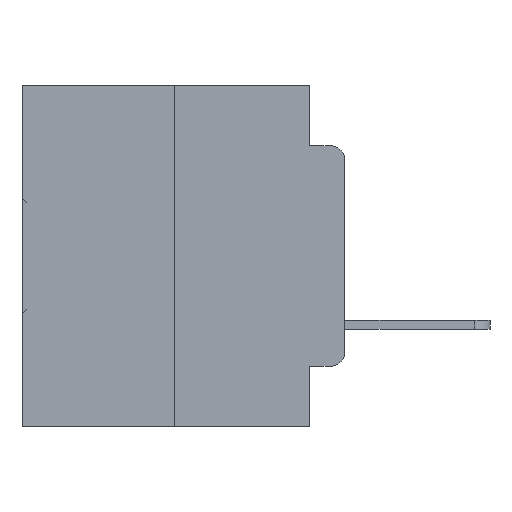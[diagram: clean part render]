
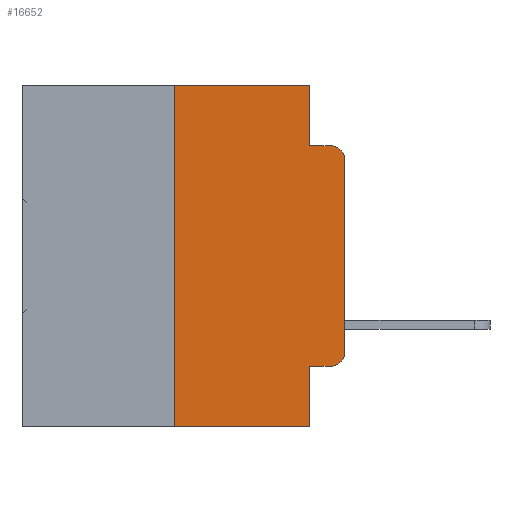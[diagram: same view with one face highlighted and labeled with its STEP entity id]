
A CAD part, left-side view. The second image highlights one B-rep face of the part: STEP entity #16652.
In plain terms, the highlighted planar face has unit normal (-1, 0, 0).
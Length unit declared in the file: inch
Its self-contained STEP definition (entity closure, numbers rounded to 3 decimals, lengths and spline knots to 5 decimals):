
#657 = AXIS2_PLACEMENT_3D ( 'NONE', #22815, #7320, #25339 ) ;
#682 = CARTESIAN_POINT ( 'NONE',  ( 0., 0., -0.1085 ) ) ;
#2944 = DIRECTION ( 'NONE',  ( 0., 0., -1. ) ) ;
#2986 = CARTESIAN_POINT ( 'NONE',  ( 0., 0.473, -0.5 ) ) ;
#3267 = VERTEX_POINT ( 'NONE', #15099 ) ;
#3400 = CARTESIAN_POINT ( 'NONE',  ( 0., 0.25, 0. ) ) ;
#3651 = ORIENTED_EDGE ( 'NONE', *, *, #21678, .F. ) ;
#3696 = PLANE ( 'NONE',  #26915 ) ;
#4369 = VERTEX_POINT ( 'NONE', #7891 ) ;
#4534 = LINE ( 'NONE', #17505, #10753 ) ;
#5088 = CARTESIAN_POINT ( 'NONE',  ( 0., 0.02, -0.4115 ) ) ;
#5525 = LINE ( 'NONE', #22235, #31099 ) ;
#5528 = DIRECTION ( 'NONE',  ( -1., 0., 0. ) ) ;
#5953 = AXIS2_PLACEMENT_3D ( 'NONE', #21174, #5528, #23659 ) ;
#5963 = EDGE_CURVE ( 'NONE', #14228, #21181, #8022, .T. ) ;
#6671 = DIRECTION ( 'NONE',  ( 0., -1., 0. ) ) ;
#7320 = DIRECTION ( 'NONE',  ( -1., 0., 0. ) ) ;
#7891 = CARTESIAN_POINT ( 'NONE',  ( 0., 0.051, -0.0885 ) ) ;
#7897 = DIRECTION ( 'NONE',  ( 0., -1., 0. ) ) ;
#8022 = LINE ( 'NONE', #25856, #21050 ) ;
#8252 = ORIENTED_EDGE ( 'NONE', *, *, #31613, .T. ) ;
#9049 = DIRECTION ( 'NONE',  ( 1., 0., 0. ) ) ;
#9266 = CARTESIAN_POINT ( 'NONE',  ( 0., 0.25, -0.5 ) ) ;
#9885 = DIRECTION ( 'NONE',  ( 0., -1., 0. ) ) ;
#10753 = VECTOR ( 'NONE', #25058, 39.37008 ) ;
#10868 = DIRECTION ( 'NONE',  ( 0., -1., 0. ) ) ;
#10975 = VERTEX_POINT ( 'NONE', #29602 ) ;
#11304 = EDGE_CURVE ( 'NONE', #14228, #10975, #32679, .T. ) ;
#11512 = CARTESIAN_POINT ( 'NONE',  ( 0., 0.25, 0. ) ) ;
#11553 = ORIENTED_EDGE ( 'NONE', *, *, #14810, .F. ) ;
#12152 = CARTESIAN_POINT ( 'NONE',  ( 0., 0.02, -0.0885 ) ) ;
#13174 = ORIENTED_EDGE ( 'NONE', *, *, #11304, .F. ) ;
#13346 = CIRCLE ( 'NONE', #5953, 0.02 ) ;
#13399 = VECTOR ( 'NONE', #2944, 39.37008 ) ;
#14009 = DIRECTION ( 'NONE',  ( 0., 0., 1. ) ) ;
#14113 = VECTOR ( 'NONE', #10868, 39.37008 ) ;
#14228 = VERTEX_POINT ( 'NONE', #14538 ) ;
#14230 = VERTEX_POINT ( 'NONE', #9266 ) ;
#14538 = CARTESIAN_POINT ( 'NONE',  ( 0., 0.051, -0.4115 ) ) ;
#14810 = EDGE_CURVE ( 'NONE', #14230, #20760, #17217, .T. ) ;
#15099 = CARTESIAN_POINT ( 'NONE',  ( 0., 0., -0.3915 ) ) ;
#16054 = VERTEX_POINT ( 'NONE', #682 ) ;
#16482 = LINE ( 'NONE', #32558, #22415 ) ;
#16652 = ADVANCED_FACE ( 'NONE', ( #24041 ), #3696, .F. ) ;
#17217 = LINE ( 'NONE', #11512, #23117 ) ;
#17505 = CARTESIAN_POINT ( 'NONE',  ( 0., 0., 0. ) ) ;
#18045 = CARTESIAN_POINT ( 'NONE',  ( 0., 0.051, 0. ) ) ;
#18107 = EDGE_CURVE ( 'NONE', #14230, #10975, #21766, .T. ) ;
#18738 = CARTESIAN_POINT ( 'NONE',  ( 0., 0.051, 0. ) ) ;
#20091 = ORIENTED_EDGE ( 'NONE', *, *, #5963, .T. ) ;
#20760 = VERTEX_POINT ( 'NONE', #3400 ) ;
#20888 = ORIENTED_EDGE ( 'NONE', *, *, #32238, .T. ) ;
#21050 = VECTOR ( 'NONE', #7897, 39.37008 ) ;
#21174 = CARTESIAN_POINT ( 'NONE',  ( 0., 0.02, -0.1085 ) ) ;
#21181 = VERTEX_POINT ( 'NONE', #5088 ) ;
#21678 = EDGE_CURVE ( 'NONE', #22704, #4369, #29502, .T. ) ;
#21766 = LINE ( 'NONE', #2986, #14113 ) ;
#22028 = ORIENTED_EDGE ( 'NONE', *, *, #26680, .T. ) ;
#22235 = CARTESIAN_POINT ( 'NONE',  ( 0., 0.473, 0. ) ) ;
#22415 = VECTOR ( 'NONE', #9885, 39.37008 ) ;
#22645 = EDGE_LOOP ( 'NONE', ( #8252, #22028, #30132, #3651, #30898, #11553, #32468, #13174, #20091, #20888 ) ) ;
#22704 = VERTEX_POINT ( 'NONE', #24022 ) ;
#22815 = CARTESIAN_POINT ( 'NONE',  ( 0., 0.02, -0.3915 ) ) ;
#22921 = VECTOR ( 'NONE', #25594, 39.37008 ) ;
#23117 = VECTOR ( 'NONE', #14009, 39.37008 ) ;
#23659 = DIRECTION ( 'NONE',  ( 0., 0., -1. ) ) ;
#23969 = CIRCLE ( 'NONE', #657, 0.02 ) ;
#24022 = CARTESIAN_POINT ( 'NONE',  ( 0., 0.051, 0. ) ) ;
#24041 = FACE_OUTER_BOUND ( 'NONE', #22645, .T. ) ;
#24160 = VERTEX_POINT ( 'NONE', #12152 ) ;
#25032 = EDGE_CURVE ( 'NONE', #4369, #24160, #16482, .T. ) ;
#25058 = DIRECTION ( 'NONE',  ( 0., 0., 1. ) ) ;
#25339 = DIRECTION ( 'NONE',  ( 0., 0., -1. ) ) ;
#25594 = DIRECTION ( 'NONE',  ( 0., 0., -1. ) ) ;
#25856 = CARTESIAN_POINT ( 'NONE',  ( 0., 0.051, -0.4115 ) ) ;
#26295 = EDGE_CURVE ( 'NONE', #20760, #22704, #5525, .T. ) ;
#26680 = EDGE_CURVE ( 'NONE', #16054, #24160, #13346, .T. ) ;
#26915 = AXIS2_PLACEMENT_3D ( 'NONE', #31783, #9049, #26952 ) ;
#26952 = DIRECTION ( 'NONE',  ( 0., 0., -1. ) ) ;
#29502 = LINE ( 'NONE', #18045, #22921 ) ;
#29602 = CARTESIAN_POINT ( 'NONE',  ( 0., 0.051, -0.5 ) ) ;
#30132 = ORIENTED_EDGE ( 'NONE', *, *, #25032, .F. ) ;
#30898 = ORIENTED_EDGE ( 'NONE', *, *, #26295, .F. ) ;
#31099 = VECTOR ( 'NONE', #6671, 39.37008 ) ;
#31613 = EDGE_CURVE ( 'NONE', #3267, #16054, #4534, .T. ) ;
#31783 = CARTESIAN_POINT ( 'NONE',  ( 0., 0.473, 0. ) ) ;
#32238 = EDGE_CURVE ( 'NONE', #21181, #3267, #23969, .T. ) ;
#32468 = ORIENTED_EDGE ( 'NONE', *, *, #18107, .T. ) ;
#32558 = CARTESIAN_POINT ( 'NONE',  ( 0., 0.051, -0.0885 ) ) ;
#32679 = LINE ( 'NONE', #18738, #13399 ) ;
